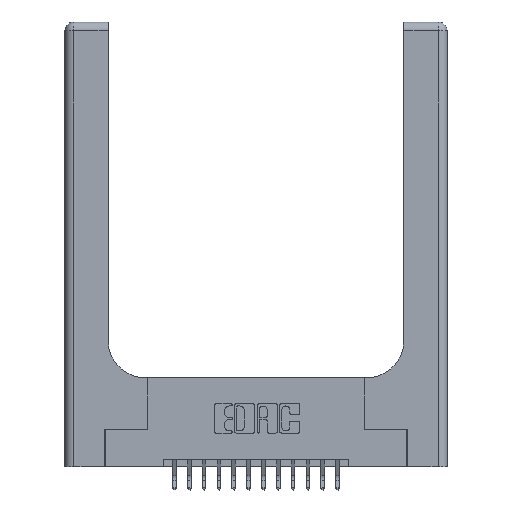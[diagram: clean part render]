
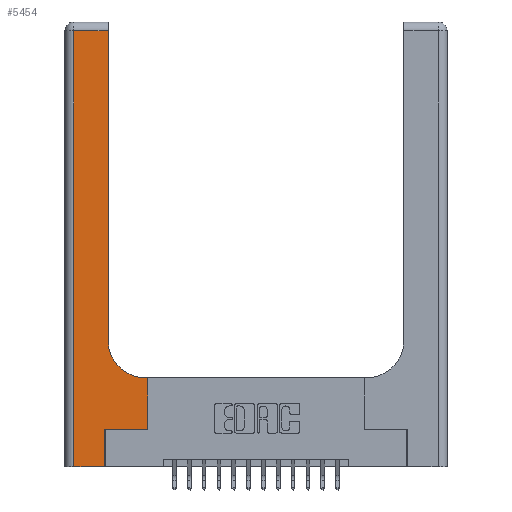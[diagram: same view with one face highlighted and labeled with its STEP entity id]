
A CAD part, top view. The second image highlights one B-rep face of the part: STEP entity #5454.
In plain terms, the highlighted planar face has unit normal (0, 0, 1).
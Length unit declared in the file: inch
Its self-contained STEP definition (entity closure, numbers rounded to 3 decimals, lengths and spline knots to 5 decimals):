
#81 = VERTEX_POINT ( 'NONE', #12756 ) ;
#744 = CARTESIAN_POINT ( 'NONE',  ( 0.269, 0., 0.37 ) ) ;
#832 = LINE ( 'NONE', #18429, #17015 ) ;
#1167 = CARTESIAN_POINT ( 'NONE',  ( 0.5415, 0.6, 0.37 ) ) ;
#1368 = LINE ( 'NONE', #744, #4549 ) ;
#2333 = DIRECTION ( 'NONE',  ( 0., 0., -1. ) ) ;
#2356 = VECTOR ( 'NONE', #12397, 39.37008 ) ;
#3290 = DIRECTION ( 'NONE',  ( -1., 0., 0. ) ) ;
#3325 = VECTOR ( 'NONE', #3290, 39.37008 ) ;
#4523 = VECTOR ( 'NONE', #16307, 39.37008 ) ;
#4549 = VECTOR ( 'NONE', #16743, 39.37008 ) ;
#4778 = DIRECTION ( 'NONE',  ( 1., 0., 0. ) ) ;
#4970 = EDGE_CURVE ( 'NONE', #12381, #12811, #11090, .T. ) ;
#4973 = VERTEX_POINT ( 'NONE', #17405 ) ;
#5094 = DIRECTION ( 'NONE',  ( 0., 1., 0. ) ) ;
#5454 = ADVANCED_FACE ( 'NONE', ( #6559 ), #18187, .F. ) ;
#5626 = ORIENTED_EDGE ( 'NONE', *, *, #16709, .T. ) ;
#5686 = ORIENTED_EDGE ( 'NONE', *, *, #9828, .T. ) ;
#6289 = VECTOR ( 'NONE', #5094, 39.37008 ) ;
#6295 = ORIENTED_EDGE ( 'NONE', *, *, #10469, .T. ) ;
#6559 = FACE_OUTER_BOUND ( 'NONE', #7639, .T. ) ;
#6578 = VERTEX_POINT ( 'NONE', #15504 ) ;
#6644 = VECTOR ( 'NONE', #14414, 39.37008 ) ;
#7233 = CARTESIAN_POINT ( 'NONE',  ( 0.5585, 0.25, 0.37 ) ) ;
#7462 = AXIS2_PLACEMENT_3D ( 'NONE', #7666, #10593, #4778 ) ;
#7639 = EDGE_LOOP ( 'NONE', ( #5626, #11698, #11482, #8768, #6295, #17005, #7663, #10283, #5686 ) ) ;
#7663 = ORIENTED_EDGE ( 'NONE', *, *, #15224, .T. ) ;
#7666 = CARTESIAN_POINT ( 'NONE',  ( 0.5415, 0.85, 0.37 ) ) ;
#7775 = LINE ( 'NONE', #17520, #9151 ) ;
#8195 = CARTESIAN_POINT ( 'NONE',  ( 0.06, 2.94, 0.37 ) ) ;
#8466 = CIRCLE ( 'NONE', #7462, 0.25 ) ;
#8768 = ORIENTED_EDGE ( 'NONE', *, *, #17458, .T. ) ;
#9113 = CARTESIAN_POINT ( 'NONE',  ( 0.2915, 0.6, 0.37 ) ) ;
#9151 = VECTOR ( 'NONE', #11716, 39.37008 ) ;
#9828 = EDGE_CURVE ( 'NONE', #12811, #4973, #8466, .T. ) ;
#10018 = CARTESIAN_POINT ( 'NONE',  ( 0.269, 0.25, 0.37 ) ) ;
#10283 = ORIENTED_EDGE ( 'NONE', *, *, #4970, .T. ) ;
#10469 = EDGE_CURVE ( 'NONE', #11360, #17424, #1368, .T. ) ;
#10593 = DIRECTION ( 'NONE',  ( 0., 0., -1. ) ) ;
#11090 = LINE ( 'NONE', #9113, #3325 ) ;
#11172 = DIRECTION ( 'NONE',  ( -1., 0., 0. ) ) ;
#11217 = LINE ( 'NONE', #12939, #6644 ) ;
#11360 = VERTEX_POINT ( 'NONE', #15078 ) ;
#11482 = ORIENTED_EDGE ( 'NONE', *, *, #18116, .T. ) ;
#11698 = ORIENTED_EDGE ( 'NONE', *, *, #13412, .T. ) ;
#11716 = DIRECTION ( 'NONE',  ( 0., -1., 0. ) ) ;
#12381 = VERTEX_POINT ( 'NONE', #13043 ) ;
#12397 = DIRECTION ( 'NONE',  ( 0., 1., 0. ) ) ;
#12552 = EDGE_CURVE ( 'NONE', #17424, #18728, #16631, .T. ) ;
#12756 = CARTESIAN_POINT ( 'NONE',  ( 0.2915, 2.94, 0.37 ) ) ;
#12811 = VERTEX_POINT ( 'NONE', #1167 ) ;
#12939 = CARTESIAN_POINT ( 'NONE',  ( 0., 0., 0.37 ) ) ;
#13043 = CARTESIAN_POINT ( 'NONE',  ( 0.5585, 0.6, 0.37 ) ) ;
#13412 = EDGE_CURVE ( 'NONE', #81, #14391, #832, .T. ) ;
#13832 = CARTESIAN_POINT ( 'NONE',  ( 0.5585, 0.25, 0.37 ) ) ;
#13963 = LINE ( 'NONE', #17824, #2356 ) ;
#14211 = AXIS2_PLACEMENT_3D ( 'NONE', #16858, #2333, #18315 ) ;
#14391 = VERTEX_POINT ( 'NONE', #8195 ) ;
#14414 = DIRECTION ( 'NONE',  ( 1., 0., 0. ) ) ;
#14666 = CARTESIAN_POINT ( 'NONE',  ( 0.269, 0.25, 0.37 ) ) ;
#15078 = CARTESIAN_POINT ( 'NONE',  ( 0.269, 0., 0.37 ) ) ;
#15167 = LINE ( 'NONE', #13832, #6289 ) ;
#15224 = EDGE_CURVE ( 'NONE', #18728, #12381, #15167, .T. ) ;
#15504 = CARTESIAN_POINT ( 'NONE',  ( 0.06, 0., 0.37 ) ) ;
#16307 = DIRECTION ( 'NONE',  ( 1., 0., 0. ) ) ;
#16631 = LINE ( 'NONE', #14666, #4523 ) ;
#16709 = EDGE_CURVE ( 'NONE', #4973, #81, #13963, .T. ) ;
#16743 = DIRECTION ( 'NONE',  ( 0., 1., 0. ) ) ;
#16858 = CARTESIAN_POINT ( 'NONE',  ( 0., 3., 0.37 ) ) ;
#17005 = ORIENTED_EDGE ( 'NONE', *, *, #12552, .T. ) ;
#17015 = VECTOR ( 'NONE', #11172, 39.37008 ) ;
#17405 = CARTESIAN_POINT ( 'NONE',  ( 0.2915, 0.85, 0.37 ) ) ;
#17424 = VERTEX_POINT ( 'NONE', #10018 ) ;
#17458 = EDGE_CURVE ( 'NONE', #6578, #11360, #11217, .T. ) ;
#17520 = CARTESIAN_POINT ( 'NONE',  ( 0.06, 3., 0.37 ) ) ;
#17824 = CARTESIAN_POINT ( 'NONE',  ( 0.2915, 3., 0.37 ) ) ;
#18116 = EDGE_CURVE ( 'NONE', #14391, #6578, #7775, .T. ) ;
#18187 = PLANE ( 'NONE',  #14211 ) ;
#18315 = DIRECTION ( 'NONE',  ( -1., 0., 0. ) ) ;
#18429 = CARTESIAN_POINT ( 'NONE',  ( 0., 2.94, 0.37 ) ) ;
#18728 = VERTEX_POINT ( 'NONE', #7233 ) ;
